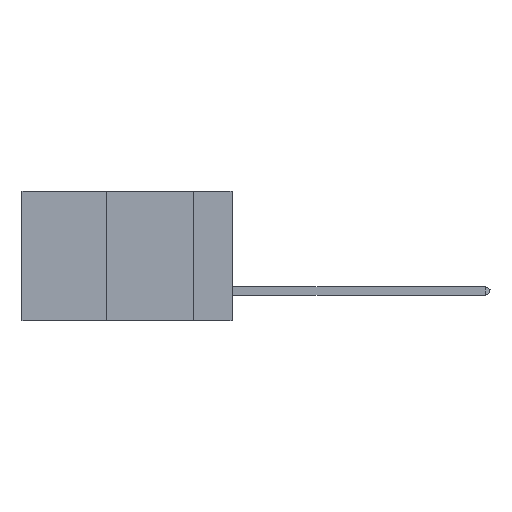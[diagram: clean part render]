
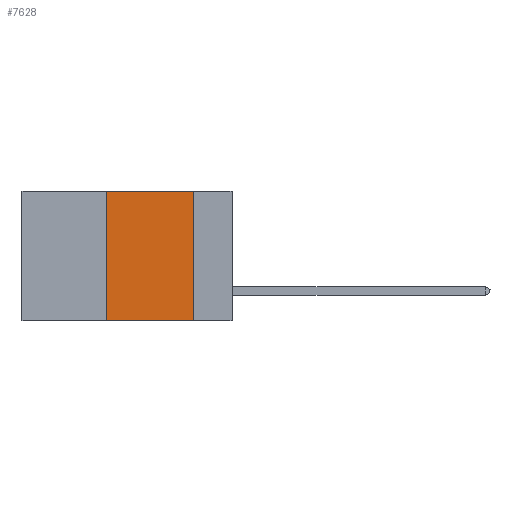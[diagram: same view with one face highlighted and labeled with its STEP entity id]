
A CAD part, left-side view. The second image highlights one B-rep face of the part: STEP entity #7628.
In plain terms, the highlighted planar face has unit normal (-1, 0, 0).
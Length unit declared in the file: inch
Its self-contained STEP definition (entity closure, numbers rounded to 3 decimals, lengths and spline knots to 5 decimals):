
#131 = LINE ( 'NONE', #13431, #5322 ) ;
#564 = FACE_OUTER_BOUND ( 'NONE', #6401, .T. ) ;
#667 = DIRECTION ( 'NONE',  ( 1., 0., 0. ) ) ;
#1912 = VECTOR ( 'NONE', #9242, 39.37008 ) ;
#2248 = LINE ( 'NONE', #5071, #1912 ) ;
#3012 = CARTESIAN_POINT ( 'NONE',  ( 0., 0.36, 0. ) ) ;
#3126 = EDGE_CURVE ( 'NONE', #4802, #3150, #2248, .T. ) ;
#3150 = VERTEX_POINT ( 'NONE', #3012 ) ;
#3722 = CARTESIAN_POINT ( 'NONE',  ( 0., 0.36, -0.37 ) ) ;
#4495 = VERTEX_POINT ( 'NONE', #13805 ) ;
#4619 = LINE ( 'NONE', #10349, #6622 ) ;
#4796 = DIRECTION ( 'NONE',  ( 0., 0., -1. ) ) ;
#4802 = VERTEX_POINT ( 'NONE', #3722 ) ;
#5071 = CARTESIAN_POINT ( 'NONE',  ( 0., 0.36, 0. ) ) ;
#5322 = VECTOR ( 'NONE', #10437, 39.37008 ) ;
#6175 = ORIENTED_EDGE ( 'NONE', *, *, #3126, .F. ) ;
#6269 = CARTESIAN_POINT ( 'NONE',  ( 0., 0.6, 0. ) ) ;
#6401 = EDGE_LOOP ( 'NONE', ( #13422, #7654, #6175, #8244 ) ) ;
#6622 = VECTOR ( 'NONE', #12358, 39.37008 ) ;
#7350 = VECTOR ( 'NONE', #9503, 39.37008 ) ;
#7628 = ADVANCED_FACE ( 'NONE', ( #564 ), #10744, .F. ) ;
#7654 = ORIENTED_EDGE ( 'NONE', *, *, #9318, .F. ) ;
#8244 = ORIENTED_EDGE ( 'NONE', *, *, #10352, .T. ) ;
#9242 = DIRECTION ( 'NONE',  ( 0., 0., 1. ) ) ;
#9318 = EDGE_CURVE ( 'NONE', #3150, #11975, #11484, .T. ) ;
#9503 = DIRECTION ( 'NONE',  ( 0., -1., 0. ) ) ;
#9885 = CARTESIAN_POINT ( 'NONE',  ( 0., 0.11, 0. ) ) ;
#10349 = CARTESIAN_POINT ( 'NONE',  ( 0., 0.11, 0. ) ) ;
#10352 = EDGE_CURVE ( 'NONE', #4802, #4495, #131, .T. ) ;
#10437 = DIRECTION ( 'NONE',  ( 0., -1., 0. ) ) ;
#10744 = PLANE ( 'NONE',  #11055 ) ;
#10801 = CARTESIAN_POINT ( 'NONE',  ( 0., 0.6, 0. ) ) ;
#11055 = AXIS2_PLACEMENT_3D ( 'NONE', #10801, #667, #4796 ) ;
#11484 = LINE ( 'NONE', #6269, #7350 ) ;
#11975 = VERTEX_POINT ( 'NONE', #9885 ) ;
#12358 = DIRECTION ( 'NONE',  ( 0., 0., -1. ) ) ;
#12843 = EDGE_CURVE ( 'NONE', #11975, #4495, #4619, .T. ) ;
#13422 = ORIENTED_EDGE ( 'NONE', *, *, #12843, .F. ) ;
#13431 = CARTESIAN_POINT ( 'NONE',  ( 0., 0.6, -0.37 ) ) ;
#13805 = CARTESIAN_POINT ( 'NONE',  ( 0., 0.11, -0.37 ) ) ;
